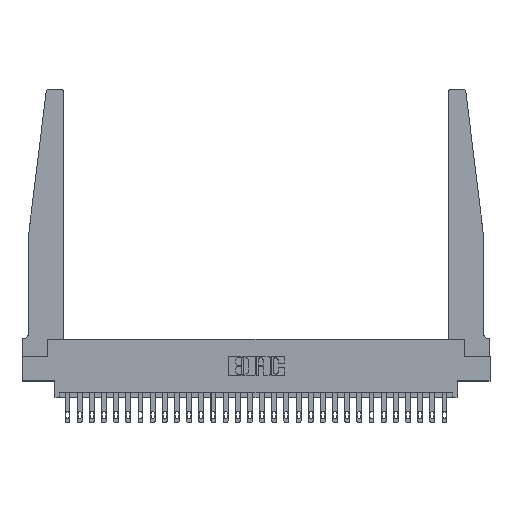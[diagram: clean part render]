
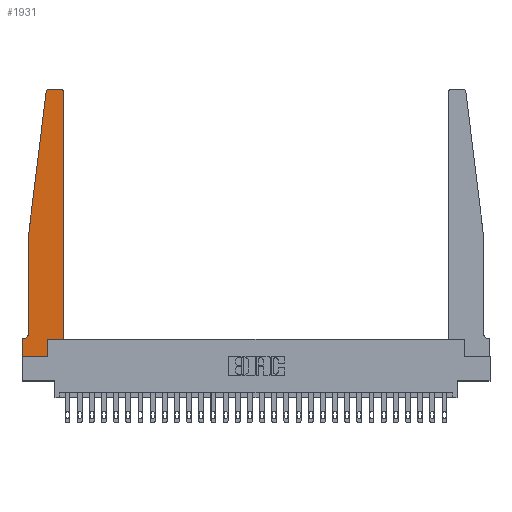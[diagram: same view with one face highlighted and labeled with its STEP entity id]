
A CAD part, top view. The second image highlights one B-rep face of the part: STEP entity #1931.
In plain terms, the highlighted planar face has unit normal (0, 0, 1).
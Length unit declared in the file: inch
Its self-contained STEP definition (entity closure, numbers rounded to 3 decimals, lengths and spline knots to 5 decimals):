
#388 = ORIENTED_EDGE ( 'NONE', *, *, #19996, .T. ) ;
#636 = VECTOR ( 'NONE', #4040, 39.37008 ) ;
#778 = DIRECTION ( 'NONE',  ( -0.122, -0.992, 0. ) ) ;
#895 = ORIENTED_EDGE ( 'NONE', *, *, #13166, .T. ) ;
#1018 = LINE ( 'NONE', #7167, #4202 ) ;
#1931 = ADVANCED_FACE ( 'NONE', ( #11608 ), #17858, .T. ) ;
#2015 = VECTOR ( 'NONE', #12540, 39.37008 ) ;
#2060 = ORIENTED_EDGE ( 'NONE', *, *, #15405, .T. ) ;
#2833 = LINE ( 'NONE', #3406, #17527 ) ;
#2882 = CARTESIAN_POINT ( 'NONE',  ( 0.065, 0.2375, 0.37 ) ) ;
#2934 = CARTESIAN_POINT ( 'NONE',  ( 0.065, 1.25, 0.37 ) ) ;
#3406 = CARTESIAN_POINT ( 'NONE',  ( 0.425, 0.18, 0.37 ) ) ;
#3758 = VECTOR ( 'NONE', #11694, 39.37008 ) ;
#4040 = DIRECTION ( 'NONE',  ( 0., -1., 0. ) ) ;
#4202 = VECTOR ( 'NONE', #17735, 39.37008 ) ;
#4486 = CARTESIAN_POINT ( 'NONE',  ( 0.425, 0.18, 0.37 ) ) ;
#4584 = ORIENTED_EDGE ( 'NONE', *, *, #7649, .T. ) ;
#4962 = VERTEX_POINT ( 'NONE', #18522 ) ;
#5184 = VERTEX_POINT ( 'NONE', #20656 ) ;
#6109 = CARTESIAN_POINT ( 'NONE',  ( 0.425, 0.18, 0.37 ) ) ;
#6150 = CARTESIAN_POINT ( 'NONE',  ( 0., 0., 0.37 ) ) ;
#6264 = LINE ( 'NONE', #10472, #2015 ) ;
#6673 = AXIS2_PLACEMENT_3D ( 'NONE', #11951, #22519, #20430 ) ;
#6989 = LINE ( 'NONE', #22135, #3758 ) ;
#7081 = DIRECTION ( 'NONE',  ( 0., 1., 0. ) ) ;
#7167 = CARTESIAN_POINT ( 'NONE',  ( 0.25, 2.75, 0.37 ) ) ;
#7196 = VERTEX_POINT ( 'NONE', #16459 ) ;
#7239 = VERTEX_POINT ( 'NONE', #25090 ) ;
#7253 = VERTEX_POINT ( 'NONE', #25359 ) ;
#7354 = CARTESIAN_POINT ( 'NONE',  ( 0.425, 2.72, 0.37 ) ) ;
#7371 = AXIS2_PLACEMENT_3D ( 'NONE', #12312, #14548, #20379 ) ;
#7520 = CARTESIAN_POINT ( 'NONE',  ( 0.24675, 2.72367, 0.37 ) ) ;
#7649 = EDGE_CURVE ( 'NONE', #9844, #7239, #21793, .T. ) ;
#9413 = EDGE_CURVE ( 'NONE', #7253, #20746, #1018, .T. ) ;
#9459 = EDGE_CURVE ( 'NONE', #21537, #7253, #18441, .T. ) ;
#9488 = LINE ( 'NONE', #2934, #9582 ) ;
#9582 = VECTOR ( 'NONE', #23936, 39.37008 ) ;
#9844 = VERTEX_POINT ( 'NONE', #7520 ) ;
#10024 = EDGE_CURVE ( 'NONE', #26005, #21537, #25438, .T. ) ;
#10472 = CARTESIAN_POINT ( 'NONE',  ( 0., 0., 0.37 ) ) ;
#10831 = CARTESIAN_POINT ( 'NONE',  ( 0.2605, 0.18, 0.37 ) ) ;
#11608 = FACE_OUTER_BOUND ( 'NONE', #25682, .T. ) ;
#11694 = DIRECTION ( 'NONE',  ( -1., 0., 0. ) ) ;
#11951 = CARTESIAN_POINT ( 'NONE',  ( 0.27653, 2.72, 0.37 ) ) ;
#12312 = CARTESIAN_POINT ( 'NONE',  ( 0.395, 2.72, 0.37 ) ) ;
#12540 = DIRECTION ( 'NONE',  ( 1., 0., 0. ) ) ;
#12790 = ORIENTED_EDGE ( 'NONE', *, *, #21897, .T. ) ;
#13166 = EDGE_CURVE ( 'NONE', #20746, #9844, #18639, .T. ) ;
#13298 = CARTESIAN_POINT ( 'NONE',  ( 0., 0.1875, 0.37 ) ) ;
#13407 = CARTESIAN_POINT ( 'NONE',  ( 0.015, 0.2375, 0.37 ) ) ;
#13433 = DIRECTION ( 'NONE',  ( 1., 0., 0. ) ) ;
#13439 = DIRECTION ( 'NONE',  ( 1., 0., 0. ) ) ;
#13547 = DIRECTION ( 'NONE',  ( -1., 0., 0. ) ) ;
#13718 = CIRCLE ( 'NONE', #16359, 0.05 ) ;
#14312 = ORIENTED_EDGE ( 'NONE', *, *, #10024, .T. ) ;
#14548 = DIRECTION ( 'NONE',  ( 0., 0., 1. ) ) ;
#14619 = DIRECTION ( 'NONE',  ( 0., 1., 0. ) ) ;
#15006 = ORIENTED_EDGE ( 'NONE', *, *, #20016, .T. ) ;
#15405 = EDGE_CURVE ( 'NONE', #26460, #26005, #2833, .T. ) ;
#15495 = DIRECTION ( 'NONE',  ( 0., 0., -1. ) ) ;
#15520 = CARTESIAN_POINT ( 'NONE',  ( 0., 0.1875, 0.37 ) ) ;
#16359 = AXIS2_PLACEMENT_3D ( 'NONE', #13407, #15495, #13547 ) ;
#16459 = CARTESIAN_POINT ( 'NONE',  ( 0.2605, 0., 0.37 ) ) ;
#16608 = VERTEX_POINT ( 'NONE', #15520 ) ;
#16921 = EDGE_CURVE ( 'NONE', #20287, #5184, #13718, .T. ) ;
#17368 = LINE ( 'NONE', #10831, #21931 ) ;
#17527 = VECTOR ( 'NONE', #13439, 39.37008 ) ;
#17735 = DIRECTION ( 'NONE',  ( -1., 0., 0. ) ) ;
#17805 = CARTESIAN_POINT ( 'NONE',  ( 0.2605, 0.18, 0.37 ) ) ;
#17858 = PLANE ( 'NONE',  #20896 ) ;
#18123 = CARTESIAN_POINT ( 'NONE',  ( 0.27653, 2.75, 0.37 ) ) ;
#18288 = ORIENTED_EDGE ( 'NONE', *, *, #20863, .T. ) ;
#18441 = CIRCLE ( 'NONE', #7371, 0.03 ) ;
#18522 = CARTESIAN_POINT ( 'NONE',  ( 0., 0., 0.37 ) ) ;
#18639 = CIRCLE ( 'NONE', #6673, 0.03 ) ;
#18953 = LINE ( 'NONE', #6150, #636 ) ;
#19861 = CARTESIAN_POINT ( 'NONE',  ( 0.065, 1.25, 0.37 ) ) ;
#19996 = EDGE_CURVE ( 'NONE', #7239, #20287, #9488, .T. ) ;
#20016 = EDGE_CURVE ( 'NONE', #5184, #16608, #6989, .T. ) ;
#20287 = VERTEX_POINT ( 'NONE', #2882 ) ;
#20379 = DIRECTION ( 'NONE',  ( 1., 0., 0. ) ) ;
#20430 = DIRECTION ( 'NONE',  ( 1., 0., 0. ) ) ;
#20656 = CARTESIAN_POINT ( 'NONE',  ( 0.015, 0.1875, 0.37 ) ) ;
#20708 = ORIENTED_EDGE ( 'NONE', *, *, #9413, .T. ) ;
#20746 = VERTEX_POINT ( 'NONE', #18123 ) ;
#20863 = EDGE_CURVE ( 'NONE', #4962, #7196, #6264, .T. ) ;
#20896 = AXIS2_PLACEMENT_3D ( 'NONE', #13298, #26215, #13433 ) ;
#21008 = ORIENTED_EDGE ( 'NONE', *, *, #9459, .T. ) ;
#21537 = VERTEX_POINT ( 'NONE', #7354 ) ;
#21793 = LINE ( 'NONE', #19861, #26893 ) ;
#21897 = EDGE_CURVE ( 'NONE', #16608, #4962, #18953, .T. ) ;
#21931 = VECTOR ( 'NONE', #7081, 39.37008 ) ;
#22135 = CARTESIAN_POINT ( 'NONE',  ( 0.065, 0.1875, 0.37 ) ) ;
#22519 = DIRECTION ( 'NONE',  ( 0., 0., 1. ) ) ;
#22706 = EDGE_CURVE ( 'NONE', #7196, #26460, #17368, .T. ) ;
#23936 = DIRECTION ( 'NONE',  ( 0., -1., 0. ) ) ;
#24550 = VECTOR ( 'NONE', #14619, 39.37008 ) ;
#25090 = CARTESIAN_POINT ( 'NONE',  ( 0.065, 1.25, 0.37 ) ) ;
#25316 = ORIENTED_EDGE ( 'NONE', *, *, #16921, .T. ) ;
#25359 = CARTESIAN_POINT ( 'NONE',  ( 0.395, 2.75, 0.37 ) ) ;
#25438 = LINE ( 'NONE', #6109, #24550 ) ;
#25682 = EDGE_LOOP ( 'NONE', ( #20708, #895, #4584, #388, #25316, #15006, #12790, #18288, #26916, #2060, #14312, #21008 ) ) ;
#26005 = VERTEX_POINT ( 'NONE', #4486 ) ;
#26215 = DIRECTION ( 'NONE',  ( 0., 0., 1. ) ) ;
#26460 = VERTEX_POINT ( 'NONE', #17805 ) ;
#26893 = VECTOR ( 'NONE', #778, 39.37008 ) ;
#26916 = ORIENTED_EDGE ( 'NONE', *, *, #22706, .T. ) ;
